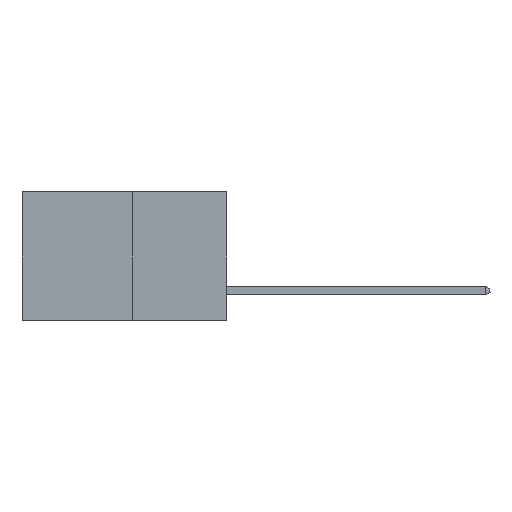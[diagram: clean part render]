
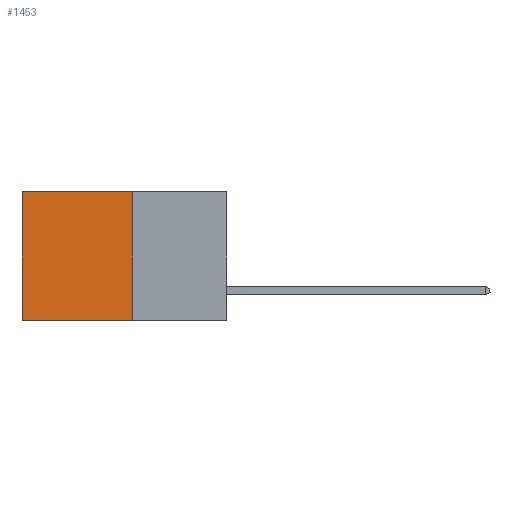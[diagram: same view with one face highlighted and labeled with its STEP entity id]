
A CAD part, left-side view. The second image highlights one B-rep face of the part: STEP entity #1453.
In plain terms, the highlighted planar face has unit normal (-1, 0, 0).
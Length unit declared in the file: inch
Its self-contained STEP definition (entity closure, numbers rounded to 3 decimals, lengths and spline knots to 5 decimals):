
#164 = VERTEX_POINT ( 'NONE', #4406 ) ;
#184 = CARTESIAN_POINT ( 'NONE',  ( 0.277, 0.59, 0. ) ) ;
#191 = EDGE_CURVE ( 'NONE', #7539, #13547, #5721, .T. ) ;
#782 = DIRECTION ( 'NONE',  ( 0., 0., -1. ) ) ;
#1182 = ORIENTED_EDGE ( 'NONE', *, *, #14941, .F. ) ;
#1215 = PLANE ( 'NONE',  #2192 ) ;
#1320 = ORIENTED_EDGE ( 'NONE', *, *, #6142, .F. ) ;
#1453 = ADVANCED_FACE ( 'NONE', ( #7453 ), #1215, .F. ) ;
#1516 = ORIENTED_EDGE ( 'NONE', *, *, #4004, .T. ) ;
#2192 = AXIS2_PLACEMENT_3D ( 'NONE', #8722, #8769, #782 ) ;
#2930 = ORIENTED_EDGE ( 'NONE', *, *, #191, .T. ) ;
#3157 = VECTOR ( 'NONE', #9609, 39.37008 ) ;
#3518 = CARTESIAN_POINT ( 'NONE',  ( 0.277, 0.59, -0.37 ) ) ;
#3692 = CARTESIAN_POINT ( 'NONE',  ( 0.277, 0.27, -0.37 ) ) ;
#4004 = EDGE_CURVE ( 'NONE', #15431, #7539, #16585, .T. ) ;
#4406 = CARTESIAN_POINT ( 'NONE',  ( 0.277, 0.27, -0.37 ) ) ;
#5309 = DIRECTION ( 'NONE',  ( 0., 1., 0. ) ) ;
#5394 = CARTESIAN_POINT ( 'NONE',  ( 0.277, 0.59, -0.37 ) ) ;
#5721 = LINE ( 'NONE', #5394, #15665 ) ;
#6142 = EDGE_CURVE ( 'NONE', #164, #13547, #13777, .T. ) ;
#6616 = CARTESIAN_POINT ( 'NONE',  ( 0.277, 0.27, -0.37 ) ) ;
#6844 = DIRECTION ( 'NONE',  ( 0., 0., -1. ) ) ;
#6862 = LINE ( 'NONE', #3692, #9933 ) ;
#7453 = FACE_OUTER_BOUND ( 'NONE', #16704, .T. ) ;
#7539 = VERTEX_POINT ( 'NONE', #184 ) ;
#8296 = CARTESIAN_POINT ( 'NONE',  ( 0.277, 0.27, 0. ) ) ;
#8722 = CARTESIAN_POINT ( 'NONE',  ( 0.277, 0.27, -0.37 ) ) ;
#8723 = CARTESIAN_POINT ( 'NONE',  ( 0.277, 0.27, 0. ) ) ;
#8769 = DIRECTION ( 'NONE',  ( 1., 0., 0. ) ) ;
#9609 = DIRECTION ( 'NONE',  ( 0., 1., 0. ) ) ;
#9933 = VECTOR ( 'NONE', #10282, 39.37008 ) ;
#10282 = DIRECTION ( 'NONE',  ( 0., 0., -1. ) ) ;
#10332 = VECTOR ( 'NONE', #5309, 39.37008 ) ;
#13547 = VERTEX_POINT ( 'NONE', #3518 ) ;
#13777 = LINE ( 'NONE', #6616, #10332 ) ;
#14941 = EDGE_CURVE ( 'NONE', #15431, #164, #6862, .T. ) ;
#15431 = VERTEX_POINT ( 'NONE', #8723 ) ;
#15665 = VECTOR ( 'NONE', #6844, 39.37008 ) ;
#16585 = LINE ( 'NONE', #8296, #3157 ) ;
#16704 = EDGE_LOOP ( 'NONE', ( #2930, #1320, #1182, #1516 ) ) ;
